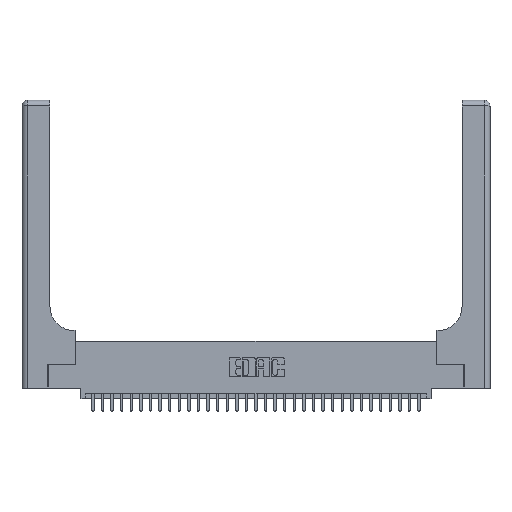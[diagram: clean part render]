
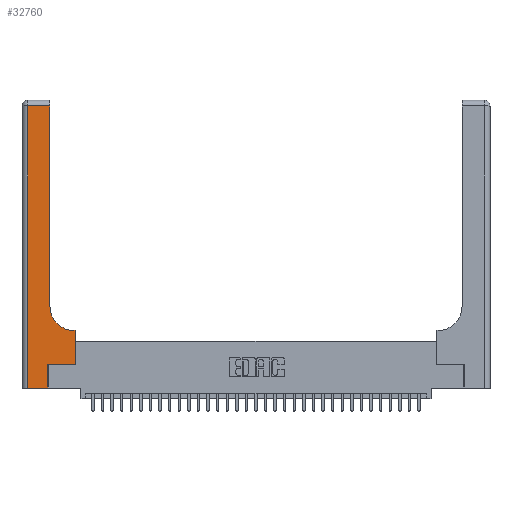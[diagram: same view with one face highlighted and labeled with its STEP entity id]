
A CAD part, top view. The second image highlights one B-rep face of the part: STEP entity #32760.
In plain terms, the highlighted planar face has unit normal (0, 0, 1).
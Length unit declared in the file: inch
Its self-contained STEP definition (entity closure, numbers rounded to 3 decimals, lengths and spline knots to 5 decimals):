
#174 = VECTOR ( 'NONE', #32263, 39.37008 ) ;
#1170 = VECTOR ( 'NONE', #20882, 39.37008 ) ;
#1175 = EDGE_CURVE ( 'NONE', #25072, #27308, #15098, .T. ) ;
#1273 = DIRECTION ( 'NONE',  ( -1., 0., 0. ) ) ;
#2377 = VECTOR ( 'NONE', #26394, 39.37008 ) ;
#3121 = VERTEX_POINT ( 'NONE', #22233 ) ;
#3198 = EDGE_CURVE ( 'NONE', #3121, #19024, #32544, .T. ) ;
#4498 = EDGE_CURVE ( 'NONE', #26818, #3121, #19875, .T. ) ;
#4544 = DIRECTION ( 'NONE',  ( -1., 0., 0. ) ) ;
#4682 = DIRECTION ( 'NONE',  ( 1., 0., 0. ) ) ;
#5894 = VECTOR ( 'NONE', #19323, 39.37008 ) ;
#5949 = ORIENTED_EDGE ( 'NONE', *, *, #23618, .T. ) ;
#6533 = DIRECTION ( 'NONE',  ( 1., 0., 0. ) ) ;
#8393 = ORIENTED_EDGE ( 'NONE', *, *, #32726, .T. ) ;
#9545 = DIRECTION ( 'NONE',  ( 0., 0., -1. ) ) ;
#10670 = ORIENTED_EDGE ( 'NONE', *, *, #18141, .T. ) ;
#10698 = LINE ( 'NONE', #32597, #23769 ) ;
#14341 = ORIENTED_EDGE ( 'NONE', *, *, #22470, .T. ) ;
#14459 = CARTESIAN_POINT ( 'NONE',  ( 0., 0., 0.37 ) ) ;
#14906 = CIRCLE ( 'NONE', #30517, 0.25 ) ;
#15098 = LINE ( 'NONE', #22509, #22439 ) ;
#15701 = ORIENTED_EDGE ( 'NONE', *, *, #1175, .T. ) ;
#16791 = CARTESIAN_POINT ( 'NONE',  ( 0.2915, 3., 0.37 ) ) ;
#17256 = CARTESIAN_POINT ( 'NONE',  ( 0.5585, 0.25, 0.37 ) ) ;
#17294 = CARTESIAN_POINT ( 'NONE',  ( 0., 3., 0.37 ) ) ;
#17521 = DIRECTION ( 'NONE',  ( 0., 0., -1. ) ) ;
#17867 = CARTESIAN_POINT ( 'NONE',  ( 0.5415, 0.6, 0.37 ) ) ;
#18086 = ORIENTED_EDGE ( 'NONE', *, *, #4498, .T. ) ;
#18141 = EDGE_CURVE ( 'NONE', #23286, #27909, #14906, .T. ) ;
#19024 = VERTEX_POINT ( 'NONE', #22112 ) ;
#19196 = CARTESIAN_POINT ( 'NONE',  ( 0.2915, 2.94, 0.37 ) ) ;
#19323 = DIRECTION ( 'NONE',  ( 0., 1., 0. ) ) ;
#19875 = LINE ( 'NONE', #31296, #2377 ) ;
#20882 = DIRECTION ( 'NONE',  ( 0., -1., 0. ) ) ;
#20913 = VERTEX_POINT ( 'NONE', #29091 ) ;
#20941 = LINE ( 'NONE', #29230, #174 ) ;
#21786 = EDGE_CURVE ( 'NONE', #27909, #26818, #25047, .T. ) ;
#21871 = AXIS2_PLACEMENT_3D ( 'NONE', #17294, #17521, #4544 ) ;
#22112 = CARTESIAN_POINT ( 'NONE',  ( 0.06, 0., 0.37 ) ) ;
#22233 = CARTESIAN_POINT ( 'NONE',  ( 0.06, 2.94, 0.37 ) ) ;
#22244 = CARTESIAN_POINT ( 'NONE',  ( 0.5585, 0.6, 0.37 ) ) ;
#22439 = VECTOR ( 'NONE', #6533, 39.37008 ) ;
#22470 = EDGE_CURVE ( 'NONE', #20913, #25072, #20941, .T. ) ;
#22509 = CARTESIAN_POINT ( 'NONE',  ( 0.269, 0.25, 0.37 ) ) ;
#23084 = CARTESIAN_POINT ( 'NONE',  ( 0.5585, 0.25, 0.37 ) ) ;
#23142 = ORIENTED_EDGE ( 'NONE', *, *, #21786, .T. ) ;
#23220 = ORIENTED_EDGE ( 'NONE', *, *, #3198, .T. ) ;
#23286 = VERTEX_POINT ( 'NONE', #17867 ) ;
#23618 = EDGE_CURVE ( 'NONE', #27308, #32148, #24151, .T. ) ;
#23769 = VECTOR ( 'NONE', #1273, 39.37008 ) ;
#24001 = FACE_OUTER_BOUND ( 'NONE', #30405, .T. ) ;
#24151 = LINE ( 'NONE', #17256, #30281 ) ;
#24853 = CARTESIAN_POINT ( 'NONE',  ( 0.2915, 0.85, 0.37 ) ) ;
#25047 = LINE ( 'NONE', #16791, #5894 ) ;
#25072 = VERTEX_POINT ( 'NONE', #29498 ) ;
#25185 = CARTESIAN_POINT ( 'NONE',  ( 0.5415, 0.85, 0.37 ) ) ;
#25398 = PLANE ( 'NONE',  #21871 ) ;
#26394 = DIRECTION ( 'NONE',  ( -1., 0., 0. ) ) ;
#26475 = VECTOR ( 'NONE', #30543, 39.37008 ) ;
#26818 = VERTEX_POINT ( 'NONE', #19196 ) ;
#27308 = VERTEX_POINT ( 'NONE', #23084 ) ;
#27909 = VERTEX_POINT ( 'NONE', #24853 ) ;
#29091 = CARTESIAN_POINT ( 'NONE',  ( 0.269, 0., 0.37 ) ) ;
#29230 = CARTESIAN_POINT ( 'NONE',  ( 0.269, 0., 0.37 ) ) ;
#29498 = CARTESIAN_POINT ( 'NONE',  ( 0.269, 0.25, 0.37 ) ) ;
#30278 = DIRECTION ( 'NONE',  ( 0., 1., 0. ) ) ;
#30280 = EDGE_CURVE ( 'NONE', #32148, #23286, #10698, .T. ) ;
#30281 = VECTOR ( 'NONE', #30278, 39.37008 ) ;
#30405 = EDGE_LOOP ( 'NONE', ( #23142, #18086, #23220, #8393, #14341, #15701, #5949, #33743, #10670 ) ) ;
#30517 = AXIS2_PLACEMENT_3D ( 'NONE', #25185, #9545, #4682 ) ;
#30543 = DIRECTION ( 'NONE',  ( 1., 0., 0. ) ) ;
#30949 = LINE ( 'NONE', #14459, #26475 ) ;
#31296 = CARTESIAN_POINT ( 'NONE',  ( 0., 2.94, 0.37 ) ) ;
#32148 = VERTEX_POINT ( 'NONE', #22244 ) ;
#32263 = DIRECTION ( 'NONE',  ( 0., 1., 0. ) ) ;
#32544 = LINE ( 'NONE', #33562, #1170 ) ;
#32597 = CARTESIAN_POINT ( 'NONE',  ( 0.2915, 0.6, 0.37 ) ) ;
#32726 = EDGE_CURVE ( 'NONE', #19024, #20913, #30949, .T. ) ;
#32760 = ADVANCED_FACE ( 'NONE', ( #24001 ), #25398, .F. ) ;
#33562 = CARTESIAN_POINT ( 'NONE',  ( 0.06, 3., 0.37 ) ) ;
#33743 = ORIENTED_EDGE ( 'NONE', *, *, #30280, .T. ) ;
